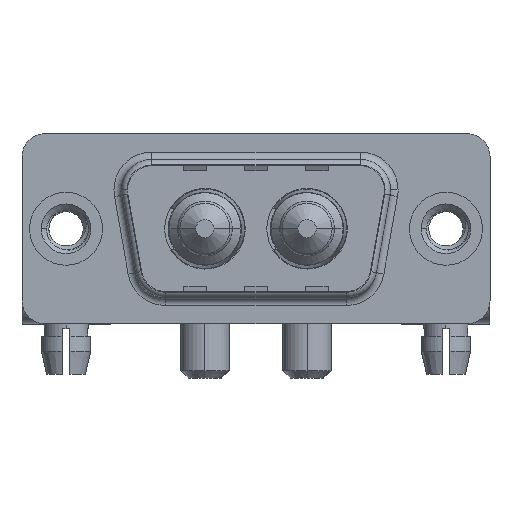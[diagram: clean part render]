
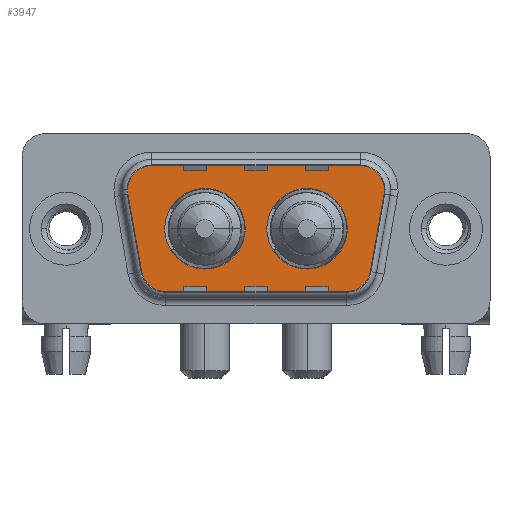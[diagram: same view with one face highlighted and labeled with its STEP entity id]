
A CAD part, top view. The second image highlights one B-rep face of the part: STEP entity #3947.
In plain terms, the highlighted planar face has unit normal (0, 0, 1).
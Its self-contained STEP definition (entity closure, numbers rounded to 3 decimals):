
#68 = EDGE_CURVE ( 'NONE', #9516, #7913, #4240, .T. ) ;
#69 = FACE_OUTER_BOUND ( 'NONE', #2419, .T. ) ;
#289 = DIRECTION ( 'NONE',  ( -1., 0., 0. ) ) ;
#380 = ORIENTED_EDGE ( 'NONE', *, *, #2118, .T. ) ;
#786 = DIRECTION ( 'NONE',  ( 0., 0., 1. ) ) ;
#791 = VERTEX_POINT ( 'NONE', #2481 ) ;
#901 = AXIS2_PLACEMENT_3D ( 'NONE', #11075, #9673, #289 ) ;
#932 = DIRECTION ( 'NONE',  ( 0.174, -0.985, 0. ) ) ;
#1003 = CARTESIAN_POINT ( 'NONE',  ( 19.564, 4.9, 0. ) ) ;
#1141 = VERTEX_POINT ( 'NONE', #14044 ) ;
#1183 = VERTEX_POINT ( 'NONE', #7899 ) ;
#1249 = EDGE_LOOP ( 'NONE', ( #11955, #1737 ) ) ;
#1275 = CARTESIAN_POINT ( 'NONE',  ( 6.459, -4.9, 0. ) ) ;
#1365 = VERTEX_POINT ( 'NONE', #5491 ) ;
#1737 = ORIENTED_EDGE ( 'NONE', *, *, #5470, .F. ) ;
#1768 = CARTESIAN_POINT ( 'NONE',  ( 21.564, 2.9, 0. ) ) ;
#2040 = CIRCLE ( 'NONE', #901, 2. ) ;
#2074 = DIRECTION ( 'NONE',  ( 0., 0., 1. ) ) ;
#2094 = AXIS2_PLACEMENT_3D ( 'NONE', #12618, #6089, #10266 ) ;
#2118 = EDGE_CURVE ( 'NONE', #1141, #791, #11302, .T. ) ;
#2218 = DIRECTION ( 'NONE',  ( 0., 0., 1. ) ) ;
#2419 = EDGE_LOOP ( 'NONE', ( #6729, #380, #9350, #3643, #13783, #10240, #9354, #12954, #9511 ) ) ;
#2481 = CARTESIAN_POINT ( 'NONE',  ( 21.534, 2.553, 0. ) ) ;
#2714 = CARTESIAN_POINT ( 'NONE',  ( 15.86, 0., 0. ) ) ;
#3116 = VERTEX_POINT ( 'NONE', #1768 ) ;
#3457 = VECTOR ( 'NONE', #932, 1000. ) ;
#3487 = VERTEX_POINT ( 'NONE', #7574 ) ;
#3543 = EDGE_CURVE ( 'NONE', #7885, #3487, #8843, .T. ) ;
#3569 = ORIENTED_EDGE ( 'NONE', *, *, #8892, .F. ) ;
#3641 = DIRECTION ( 'NONE',  ( 1., 0., 0. ) ) ;
#3643 = ORIENTED_EDGE ( 'NONE', *, *, #13370, .T. ) ;
#3671 = VECTOR ( 'NONE', #9296, 1000. ) ;
#3947 = ADVANCED_FACE ( 'NONE', ( #5388, #9987, #69 ), #7862, .T. ) ;
#4172 = CARTESIAN_POINT ( 'NONE',  ( 9.14, 0., 0. ) ) ;
#4180 = AXIS2_PLACEMENT_3D ( 'NONE', #12454, #9574, #11384 ) ;
#4240 = LINE ( 'NONE', #9924, #3457 ) ;
#4301 = CIRCLE ( 'NONE', #11793, 2.65 ) ;
#5188 = EDGE_CURVE ( 'NONE', #1365, #1183, #14092, .T. ) ;
#5388 = FACE_BOUND ( 'NONE', #1249, .T. ) ;
#5414 = VERTEX_POINT ( 'NONE', #6095 ) ;
#5440 = DIRECTION ( 'NONE',  ( -1., 0., 0. ) ) ;
#5448 = DIRECTION ( 'NONE',  ( 1., 0., 0. ) ) ;
#5470 = EDGE_CURVE ( 'NONE', #1183, #1365, #4301, .T. ) ;
#5491 = CARTESIAN_POINT ( 'NONE',  ( 18.51, 0., 0. ) ) ;
#5744 = CIRCLE ( 'NONE', #8476, 2.65 ) ;
#5827 = CARTESIAN_POINT ( 'NONE',  ( 6.49, 0., 0. ) ) ;
#5904 = AXIS2_PLACEMENT_3D ( 'NONE', #13792, #2074, #6465 ) ;
#5949 = DIRECTION ( 'NONE',  ( 0., 0., 1. ) ) ;
#6089 = DIRECTION ( 'NONE',  ( 0., 0., 1. ) ) ;
#6095 = CARTESIAN_POINT ( 'NONE',  ( 11.79, 0., 0. ) ) ;
#6164 = DIRECTION ( 'NONE',  ( 1., 0., 0. ) ) ;
#6210 = CIRCLE ( 'NONE', #7771, 2. ) ;
#6465 = DIRECTION ( 'NONE',  ( 1., 0., 0. ) ) ;
#6596 = CARTESIAN_POINT ( 'NONE',  ( 18.541, -2.9, 0. ) ) ;
#6729 = ORIENTED_EDGE ( 'NONE', *, *, #10350, .T. ) ;
#6764 = LINE ( 'NONE', #9022, #7570 ) ;
#7561 = EDGE_CURVE ( 'NONE', #791, #3116, #2040, .T. ) ;
#7570 = VECTOR ( 'NONE', #12226, 1000. ) ;
#7574 = CARTESIAN_POINT ( 'NONE',  ( 5.436, 4.9, 0. ) ) ;
#7771 = AXIS2_PLACEMENT_3D ( 'NONE', #12757, #12844, #10843 ) ;
#7862 = PLANE ( 'NONE',  #8293 ) ;
#7885 = VERTEX_POINT ( 'NONE', #1003 ) ;
#7899 = CARTESIAN_POINT ( 'NONE',  ( 13.21, 0., 0. ) ) ;
#7913 = VERTEX_POINT ( 'NONE', #9705 ) ;
#8103 = VERTEX_POINT ( 'NONE', #1275 ) ;
#8238 = DIRECTION ( 'NONE',  ( 0., 0., 1. ) ) ;
#8293 = AXIS2_PLACEMENT_3D ( 'NONE', #6596, #2218, #5448 ) ;
#8363 = DIRECTION ( 'NONE',  ( 0., 0., 1. ) ) ;
#8476 = AXIS2_PLACEMENT_3D ( 'NONE', #4172, #8238, #10379 ) ;
#8785 = CARTESIAN_POINT ( 'NONE',  ( 5.436, 4.9, 0. ) ) ;
#8843 = LINE ( 'NONE', #8785, #12372 ) ;
#8892 = EDGE_CURVE ( 'NONE', #9316, #5414, #5744, .T. ) ;
#9022 = CARTESIAN_POINT ( 'NONE',  ( 6.459, -4.9, 0. ) ) ;
#9296 = DIRECTION ( 'NONE',  ( 0.174, 0.985, 0. ) ) ;
#9316 = VERTEX_POINT ( 'NONE', #5827 ) ;
#9350 = ORIENTED_EDGE ( 'NONE', *, *, #7561, .T. ) ;
#9354 = ORIENTED_EDGE ( 'NONE', *, *, #68, .T. ) ;
#9511 = ORIENTED_EDGE ( 'NONE', *, *, #13877, .T. ) ;
#9516 = VERTEX_POINT ( 'NONE', #11709 ) ;
#9574 = DIRECTION ( 'NONE',  ( 0., 0., 1. ) ) ;
#9673 = DIRECTION ( 'NONE',  ( 0., 0., 1. ) ) ;
#9705 = CARTESIAN_POINT ( 'NONE',  ( 4.489, -3.247, 0. ) ) ;
#9906 = EDGE_CURVE ( 'NONE', #5414, #9316, #13032, .T. ) ;
#9924 = CARTESIAN_POINT ( 'NONE',  ( 3.466, 2.553, 0. ) ) ;
#9987 = FACE_BOUND ( 'NONE', #13646, .T. ) ;
#10061 = CIRCLE ( 'NONE', #13937, 2. ) ;
#10240 = ORIENTED_EDGE ( 'NONE', *, *, #10824, .T. ) ;
#10266 = DIRECTION ( 'NONE',  ( 1., 0., 0. ) ) ;
#10350 = EDGE_CURVE ( 'NONE', #10445, #1141, #13271, .T. ) ;
#10379 = DIRECTION ( 'NONE',  ( 1., 0., 0. ) ) ;
#10445 = VERTEX_POINT ( 'NONE', #11647 ) ;
#10507 = CARTESIAN_POINT ( 'NONE',  ( 21.534, 2.553, 0. ) ) ;
#10564 = CARTESIAN_POINT ( 'NONE',  ( 6.459, -2.9, 0. ) ) ;
#10824 = EDGE_CURVE ( 'NONE', #3487, #9516, #10061, .T. ) ;
#10843 = DIRECTION ( 'NONE',  ( -1., 0., 0. ) ) ;
#10992 = CIRCLE ( 'NONE', #12354, 2. ) ;
#11075 = CARTESIAN_POINT ( 'NONE',  ( 19.564, 2.9, 0. ) ) ;
#11302 = LINE ( 'NONE', #10507, #3671 ) ;
#11315 = DIRECTION ( 'NONE',  ( -1., 0., 0. ) ) ;
#11342 = EDGE_CURVE ( 'NONE', #7913, #8103, #10992, .T. ) ;
#11384 = DIRECTION ( 'NONE',  ( 1., 0., 0. ) ) ;
#11647 = CARTESIAN_POINT ( 'NONE',  ( 18.541, -4.9, 0. ) ) ;
#11709 = CARTESIAN_POINT ( 'NONE',  ( 3.466, 2.553, 0. ) ) ;
#11793 = AXIS2_PLACEMENT_3D ( 'NONE', #2714, #5949, #3641 ) ;
#11955 = ORIENTED_EDGE ( 'NONE', *, *, #5188, .F. ) ;
#12226 = DIRECTION ( 'NONE',  ( 1., 0., 0. ) ) ;
#12354 = AXIS2_PLACEMENT_3D ( 'NONE', #10564, #786, #5440 ) ;
#12372 = VECTOR ( 'NONE', #11315, 1000. ) ;
#12454 = CARTESIAN_POINT ( 'NONE',  ( 18.541, -2.9, 0. ) ) ;
#12618 = CARTESIAN_POINT ( 'NONE',  ( 9.14, 0., 0. ) ) ;
#12757 = CARTESIAN_POINT ( 'NONE',  ( 19.564, 2.9, 0. ) ) ;
#12844 = DIRECTION ( 'NONE',  ( 0., 0., 1. ) ) ;
#12954 = ORIENTED_EDGE ( 'NONE', *, *, #11342, .T. ) ;
#13032 = CIRCLE ( 'NONE', #2094, 2.65 ) ;
#13271 = CIRCLE ( 'NONE', #4180, 2. ) ;
#13370 = EDGE_CURVE ( 'NONE', #3116, #7885, #6210, .T. ) ;
#13646 = EDGE_LOOP ( 'NONE', ( #14043, #3569 ) ) ;
#13783 = ORIENTED_EDGE ( 'NONE', *, *, #3543, .T. ) ;
#13792 = CARTESIAN_POINT ( 'NONE',  ( 15.86, 0., 0. ) ) ;
#13841 = CARTESIAN_POINT ( 'NONE',  ( 5.436, 2.9, 0. ) ) ;
#13877 = EDGE_CURVE ( 'NONE', #8103, #10445, #6764, .T. ) ;
#13937 = AXIS2_PLACEMENT_3D ( 'NONE', #13841, #8363, #6164 ) ;
#14043 = ORIENTED_EDGE ( 'NONE', *, *, #9906, .F. ) ;
#14044 = CARTESIAN_POINT ( 'NONE',  ( 20.511, -3.247, 0. ) ) ;
#14092 = CIRCLE ( 'NONE', #5904, 2.65 ) ;
